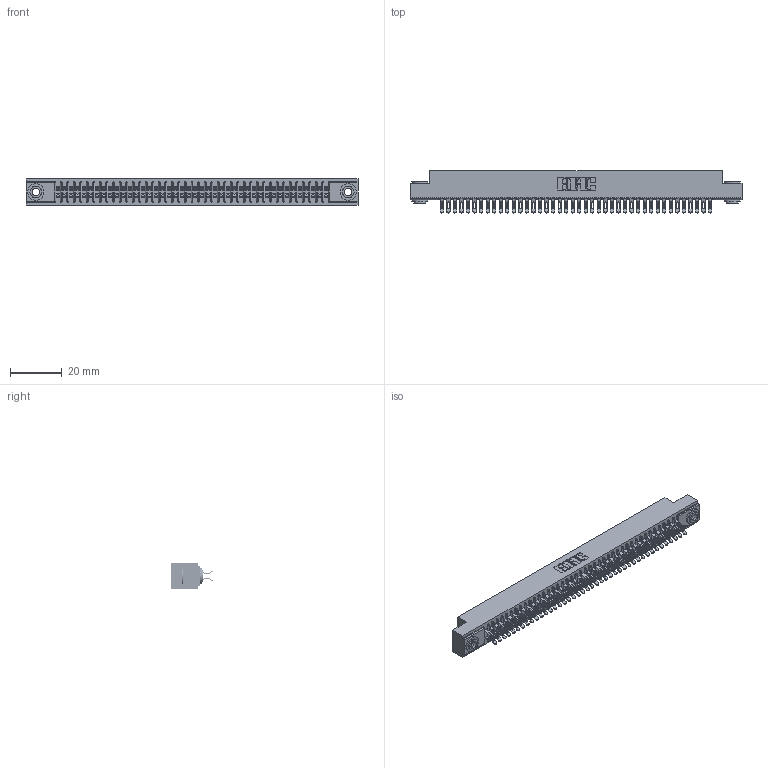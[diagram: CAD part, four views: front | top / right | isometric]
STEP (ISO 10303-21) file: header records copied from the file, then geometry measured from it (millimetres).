
FILE_DESCRIPTION (( 'STEP AP203' ), '1' );
FILE_NAME ('391-084-555-203.STEP', '2018-08-09T16:25:45', ( '' ), ( '' ), 'SwSTEP 2.0', 'SolidWorks 2016', '' );
FILE_SCHEMA (( 'CONFIG_CONTROL_DESIGN' ));
Length unit declared in the file: inch
Products named in the file (4): 341 Part_.156 (3.96) Dia Mounting Holes; 341-292-001_341-292-155; 345-250-002_345-250-002-102; 391-084-555-203
Assembly tree (87 placements, depth 2):
  391-084-555-203
    341 Part_.156 (3.96) Dia Mounting Holes
    341-292-001_341-292-155  x84
    345-250-002_345-250-002-102  x2
Bounding box: 128.91 x 16.31 x 10.16 mm (x, y, z)
Volume: 9627 mm3; surface area: 18019 mm2
Topology: 87 solids, 87 shells, 6720 faces, 20042 edges, 13046 vertices
Faces by surface type: plane 3620, cylinder 2924, sphere 86, torus 82, cone 8
Entity records: 52364 total; most frequent: CARTESIAN_POINT 8701, ORIENTED_EDGE 8628, DIRECTION 8450, EDGE_CURVE 4314, VECTOR 3460, LINE 3460, VERTEX_POINT 2730, AXIS2_PLACEMENT_3D 2495
